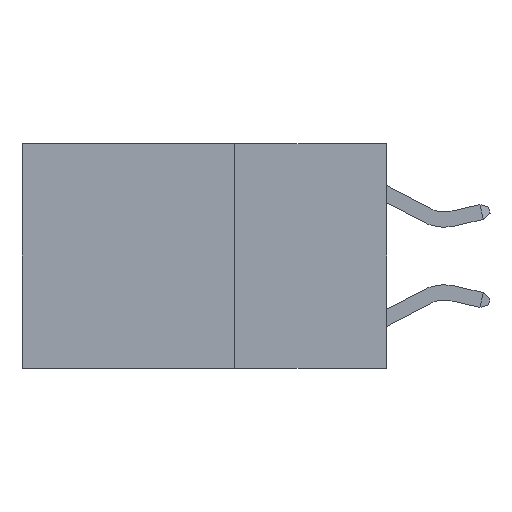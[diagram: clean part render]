
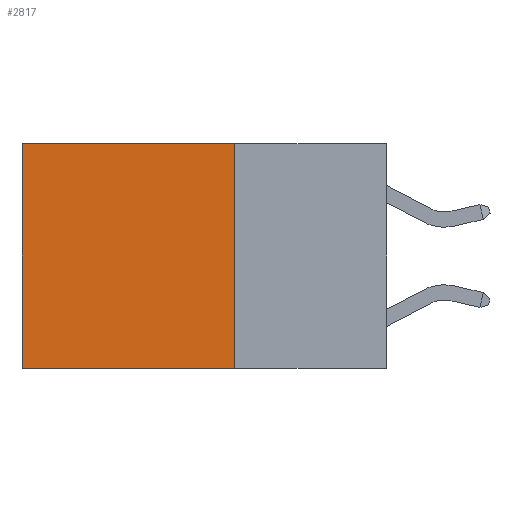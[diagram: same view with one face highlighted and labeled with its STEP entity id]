
A CAD part, left-side view. The second image highlights one B-rep face of the part: STEP entity #2817.
In plain terms, the highlighted planar face has unit normal (-1, 0, 0).
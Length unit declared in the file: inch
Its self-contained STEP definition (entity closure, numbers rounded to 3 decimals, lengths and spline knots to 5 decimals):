
#75 = CARTESIAN_POINT ( 'NONE',  ( 0.2625, 0.25, 0. ) ) ;
#343 = LINE ( 'NONE', #2070, #8863 ) ;
#908 = LINE ( 'NONE', #7417, #7369 ) ;
#1997 = VERTEX_POINT ( 'NONE', #75 ) ;
#2070 = CARTESIAN_POINT ( 'NONE',  ( 0.2625, 0.25, 0. ) ) ;
#2136 = LINE ( 'NONE', #2975, #2392 ) ;
#2392 = VECTOR ( 'NONE', #9245, 39.37008 ) ;
#2499 = DIRECTION ( 'NONE',  ( 0., 0., -1. ) ) ;
#2559 = PLANE ( 'NONE',  #8659 ) ;
#2817 = ADVANCED_FACE ( 'NONE', ( #4978 ), #2559, .F. ) ;
#2975 = CARTESIAN_POINT ( 'NONE',  ( 0.2625, 0.25, 0. ) ) ;
#3010 = EDGE_CURVE ( 'NONE', #1997, #6554, #2136, .T. ) ;
#3123 = EDGE_LOOP ( 'NONE', ( #3578, #3902, #8081, #3426 ) ) ;
#3330 = CARTESIAN_POINT ( 'NONE',  ( 0.2625, 0.6, 0. ) ) ;
#3426 = ORIENTED_EDGE ( 'NONE', *, *, #3010, .T. ) ;
#3512 = DIRECTION ( 'NONE',  ( 1., 0., 0. ) ) ;
#3578 = ORIENTED_EDGE ( 'NONE', *, *, #9004, .T. ) ;
#3902 = ORIENTED_EDGE ( 'NONE', *, *, #5387, .F. ) ;
#3928 = VERTEX_POINT ( 'NONE', #7300 ) ;
#4978 = FACE_OUTER_BOUND ( 'NONE', #3123, .T. ) ;
#5092 = EDGE_CURVE ( 'NONE', #1997, #3928, #343, .T. ) ;
#5224 = CARTESIAN_POINT ( 'NONE',  ( 0.2625, 0.25, 0. ) ) ;
#5387 = EDGE_CURVE ( 'NONE', #3928, #8651, #6761, .T. ) ;
#6454 = CARTESIAN_POINT ( 'NONE',  ( 0.2625, 0.6, -0.37 ) ) ;
#6554 = VERTEX_POINT ( 'NONE', #3330 ) ;
#6761 = LINE ( 'NONE', #8163, #10035 ) ;
#7300 = CARTESIAN_POINT ( 'NONE',  ( 0.2625, 0.25, -0.37 ) ) ;
#7369 = VECTOR ( 'NONE', #2499, 39.37008 ) ;
#7417 = CARTESIAN_POINT ( 'NONE',  ( 0.2625, 0.6, 0. ) ) ;
#8081 = ORIENTED_EDGE ( 'NONE', *, *, #5092, .F. ) ;
#8163 = CARTESIAN_POINT ( 'NONE',  ( 0.2625, 0.25, -0.37 ) ) ;
#8651 = VERTEX_POINT ( 'NONE', #6454 ) ;
#8659 = AXIS2_PLACEMENT_3D ( 'NONE', #5224, #3512, #8929 ) ;
#8863 = VECTOR ( 'NONE', #9904, 39.37008 ) ;
#8929 = DIRECTION ( 'NONE',  ( 0., 0., -1. ) ) ;
#9004 = EDGE_CURVE ( 'NONE', #6554, #8651, #908, .T. ) ;
#9245 = DIRECTION ( 'NONE',  ( 0., 1., 0. ) ) ;
#9904 = DIRECTION ( 'NONE',  ( 0., 0., -1. ) ) ;
#10035 = VECTOR ( 'NONE', #10229, 39.37008 ) ;
#10229 = DIRECTION ( 'NONE',  ( 0., 1., 0. ) ) ;
